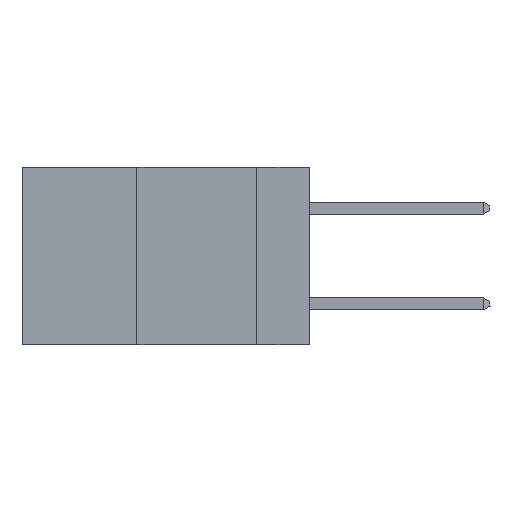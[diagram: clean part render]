
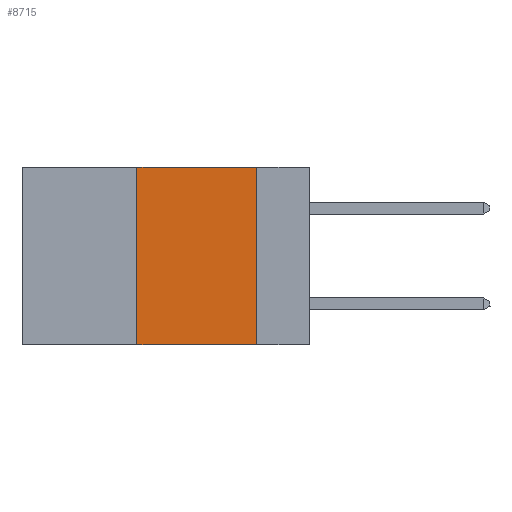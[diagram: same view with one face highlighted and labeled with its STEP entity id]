
A CAD part, left-side view. The second image highlights one B-rep face of the part: STEP entity #8715.
In plain terms, the highlighted planar face has unit normal (-1, 0, 0).
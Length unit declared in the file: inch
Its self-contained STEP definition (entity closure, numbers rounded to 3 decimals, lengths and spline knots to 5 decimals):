
#101 = EDGE_CURVE ( 'NONE', #19745, #11440, #10514, .T. ) ;
#740 = CARTESIAN_POINT ( 'NONE',  ( 0., 0.36, -0.37 ) ) ;
#1000 = CARTESIAN_POINT ( 'NONE',  ( 0., 0.11, -0.37 ) ) ;
#1309 = CARTESIAN_POINT ( 'NONE',  ( 0., 0.6, 0. ) ) ;
#1446 = DIRECTION ( 'NONE',  ( 1., 0., 0. ) ) ;
#1686 = VECTOR ( 'NONE', #19025, 39.37008 ) ;
#2106 = VERTEX_POINT ( 'NONE', #4351 ) ;
#2454 = ORIENTED_EDGE ( 'NONE', *, *, #101, .T. ) ;
#2931 = CARTESIAN_POINT ( 'NONE',  ( 0., 0.36, 0. ) ) ;
#4351 = CARTESIAN_POINT ( 'NONE',  ( 0., 0.11, 0. ) ) ;
#4953 = DIRECTION ( 'NONE',  ( 0., 0., 1. ) ) ;
#6850 = EDGE_CURVE ( 'NONE', #19745, #10550, #7324, .T. ) ;
#7324 = LINE ( 'NONE', #12168, #17725 ) ;
#8088 = VECTOR ( 'NONE', #15919, 39.37008 ) ;
#8348 = ORIENTED_EDGE ( 'NONE', *, *, #6850, .F. ) ;
#8715 = ADVANCED_FACE ( 'NONE', ( #22408 ), #15597, .F. ) ;
#10514 = LINE ( 'NONE', #13544, #8088 ) ;
#10550 = VERTEX_POINT ( 'NONE', #2931 ) ;
#10929 = EDGE_CURVE ( 'NONE', #2106, #11440, #20972, .T. ) ;
#11440 = VERTEX_POINT ( 'NONE', #1000 ) ;
#11971 = EDGE_LOOP ( 'NONE', ( #20754, #15136, #8348, #2454 ) ) ;
#12168 = CARTESIAN_POINT ( 'NONE',  ( 0., 0.36, 0. ) ) ;
#13544 = CARTESIAN_POINT ( 'NONE',  ( 0., 0.6, -0.37 ) ) ;
#14429 = DIRECTION ( 'NONE',  ( 0., 0., -1. ) ) ;
#15136 = ORIENTED_EDGE ( 'NONE', *, *, #18131, .F. ) ;
#15597 = PLANE ( 'NONE',  #21442 ) ;
#15919 = DIRECTION ( 'NONE',  ( 0., -1., 0. ) ) ;
#16226 = LINE ( 'NONE', #1309, #1686 ) ;
#16300 = VECTOR ( 'NONE', #21234, 39.37008 ) ;
#17725 = VECTOR ( 'NONE', #4953, 39.37008 ) ;
#18131 = EDGE_CURVE ( 'NONE', #10550, #2106, #16226, .T. ) ;
#19025 = DIRECTION ( 'NONE',  ( 0., -1., 0. ) ) ;
#19327 = CARTESIAN_POINT ( 'NONE',  ( 0., 0.6, 0. ) ) ;
#19745 = VERTEX_POINT ( 'NONE', #740 ) ;
#20653 = CARTESIAN_POINT ( 'NONE',  ( 0., 0.11, 0. ) ) ;
#20754 = ORIENTED_EDGE ( 'NONE', *, *, #10929, .F. ) ;
#20972 = LINE ( 'NONE', #20653, #16300 ) ;
#21234 = DIRECTION ( 'NONE',  ( 0., 0., -1. ) ) ;
#21442 = AXIS2_PLACEMENT_3D ( 'NONE', #19327, #1446, #14429 ) ;
#22408 = FACE_OUTER_BOUND ( 'NONE', #11971, .T. ) ;
